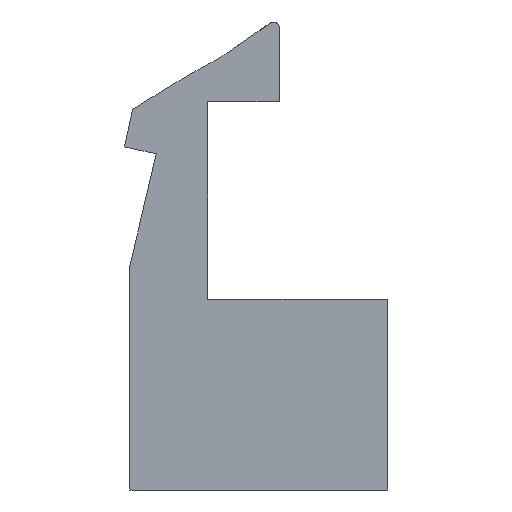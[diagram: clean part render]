
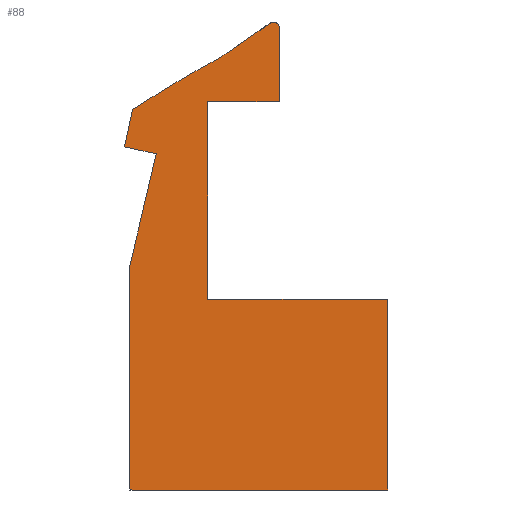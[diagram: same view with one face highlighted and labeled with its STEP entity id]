
A CAD part, front view. The second image highlights one B-rep face of the part: STEP entity #88.
In plain terms, the highlighted planar face has unit normal (0, -1, 0).
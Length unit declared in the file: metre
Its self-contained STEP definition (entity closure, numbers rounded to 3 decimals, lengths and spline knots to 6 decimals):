
#88=ADVANCED_FACE('12:6837',(#170),#171,.F.);
#170=FACE_OUTER_BOUND('',#1109,.T.);
#171=PLANE('',#1110);
#1109=EDGE_LOOP('',(#1387,#1388,#1389,#1390,#1391,#1392,#1393,#1394,#1395,#1396,#1397,#1398,#1399,#1400,#1401,#1402,#1403,#1404,#1405));
#1110=AXIS2_PLACEMENT_3D('',#1406,#1407,#1408);
#1387=ORIENTED_EDGE('',*,*,#1453,.F.);
#1388=ORIENTED_EDGE('',*,*,#1511,.T.);
#1389=ORIENTED_EDGE('',*,*,#1514,.F.);
#1390=ORIENTED_EDGE('',*,*,#1507,.F.);
#1391=ORIENTED_EDGE('',*,*,#1500,.T.);
#1392=ORIENTED_EDGE('',*,*,#1542,.F.);
#1393=ORIENTED_EDGE('',*,*,#1449,.F.);
#1394=ORIENTED_EDGE('',*,*,#1546,.F.);
#1395=ORIENTED_EDGE('',*,*,#1549,.F.);
#1396=ORIENTED_EDGE('',*,*,#1551,.F.);
#1397=ORIENTED_EDGE('',*,*,#1553,.F.);
#1398=ORIENTED_EDGE('',*,*,#1532,.F.);
#1399=ORIENTED_EDGE('',*,*,#1528,.T.);
#1400=ORIENTED_EDGE('',*,*,#1524,.F.);
#1401=ORIENTED_EDGE('',*,*,#1520,.F.);
#1402=ORIENTED_EDGE('',*,*,#1554,.F.);
#1403=ORIENTED_EDGE('',*,*,#1541,.F.);
#1404=ORIENTED_EDGE('',*,*,#1536,.T.);
#1405=ORIENTED_EDGE('',*,*,#1533,.F.);
#1406=CARTESIAN_POINT('',(0.000691,-0.01,0.018046));
#1407=DIRECTION('',(0.,1.0,0.));
#1408=DIRECTION('',(0.214,0.,0.977));
#1449=EDGE_CURVE('12:6918',#1562,#1558,#1564,.F.);
#1453=EDGE_CURVE('12:6894',#1570,#1566,#1572,.F.);
#1500=EDGE_CURVE('12:6915',#1655,#1653,#1656,.F.);
#1507=EDGE_CURVE('12:6912',#1655,#1664,#1665,.F.);
#1511=EDGE_CURVE('12:6906',#1570,#1668,#1670,.F.);
#1514=EDGE_CURVE('12:6909',#1664,#1668,#1674,.T.);
#1520=EDGE_CURVE('12:6942',#1682,#1684,#1685,.T.);
#1524=EDGE_CURVE('12:6939',#1684,#1690,#1691,.T.);
#1528=EDGE_CURVE('12:6936',#1694,#1690,#1697,.T.);
#1532=EDGE_CURVE('12:6933',#1694,#1700,#1703,.T.);
#1533=EDGE_CURVE('12:6894',#1566,#1704,#1705,.F.);
#1536=EDGE_CURVE('12:6951',#1709,#1704,#1710,.F.);
#1541=EDGE_CURVE('12:6948',#1709,#1715,#1718,.F.);
#1542=EDGE_CURVE('12:6918',#1558,#1653,#1719,.F.);
#1546=EDGE_CURVE('12:6921',#1723,#1562,#1725,.F.);
#1549=EDGE_CURVE('12:6924',#1728,#1723,#1730,.T.);
#1551=EDGE_CURVE('12:6927',#1731,#1728,#1734,.F.);
#1553=EDGE_CURVE('12:6930',#1700,#1731,#1736,.T.);
#1554=EDGE_CURVE('12:6945',#1715,#1682,#1737,.F.);
#1558=VERTEX_POINT('',#1741);
#1562=VERTEX_POINT('',#1746);
#1564=CIRCLE('',#1749,0.0535);
#1566=VERTEX_POINT('',#1751);
#1570=VERTEX_POINT('',#1756);
#1572=CIRCLE('',#1759,0.0003);
#1653=VERTEX_POINT('',#1948);
#1655=VERTEX_POINT('',#1951);
#1656=CIRCLE('',#1952,0.002);
#1664=VERTEX_POINT('',#1966);
#1665=CIRCLE('',#1967,0.006);
#1668=VERTEX_POINT('',#1972);
#1670=LINE('',#1975,#1976);
#1674=CIRCLE('',#1982,0.006);
#1682=VERTEX_POINT('',#1992);
#1684=VERTEX_POINT('',#1995);
#1685=LINE('',#1996,#1997);
#1690=VERTEX_POINT('',#2004);
#1691=LINE('',#2005,#2006);
#1694=VERTEX_POINT('',#2010);
#1697=LINE('',#2015,#2016);
#1700=VERTEX_POINT('',#2019);
#1703=LINE('',#2024,#2025);
#1704=VERTEX_POINT('',#2026);
#1705=CIRCLE('',#2027,0.0003);
#1709=VERTEX_POINT('',#2032);
#1710=LINE('',#2033,#2034);
#1715=VERTEX_POINT('',#2041);
#1718=LINE('',#2046,#2047);
#1719=CIRCLE('',#2048,0.0535);
#1723=VERTEX_POINT('',#2053);
#1725=LINE('',#2056,#2057);
#1728=VERTEX_POINT('',#2061);
#1730=LINE('',#2064,#2065);
#1731=VERTEX_POINT('',#2066);
#1734=LINE('',#2070,#2071);
#1736=LINE('',#2074,#2075);
#1737=LINE('',#2076,#2077);
#1741=CARTESIAN_POINT('',(0.002793,-0.01,0.021584));
#1746=CARTESIAN_POINT('',(0.000989,-0.01,0.020483));
#1749=AXIS2_PLACEMENT_3D('',#2087,#2088,#2089);
#1751=CARTESIAN_POINT('',(0.007659,-0.01,0.024499));
#1756=CARTESIAN_POINT('',(0.007348,-0.01,0.024479));
#1759=AXIS2_PLACEMENT_3D('',#2095,#2096,#2097);
#1948=CARTESIAN_POINT('',(0.004638,-0.01,0.022612));
#1951=CARTESIAN_POINT('',(0.004872,-0.01,0.022758));
#1952=AXIS2_PLACEMENT_3D('',#2159,#2160,#2161);
#1966=CARTESIAN_POINT('',(0.005165,-0.01,0.022957));
#1967=AXIS2_PLACEMENT_3D('',#2168,#2169,#2170);
#1972=CARTESIAN_POINT('',(0.005379,-0.01,0.0231));
#1975=CARTESIAN_POINT('',(0.003839,-0.01,0.022023));
#1976=VECTOR('',#2174,1.0);
#1982=AXIS2_PLACEMENT_3D('',#2177,#2178,#2179);
#1992=CARTESIAN_POINT('',(0.004069,-0.01,0.01));
#1995=CARTESIAN_POINT('',(0.0135,-0.01,0.01));
#1996=CARTESIAN_POINT('',(0.005,-0.01,0.01));
#1997=VECTOR('',#2189,1.0);
#2004=CARTESIAN_POINT('',(0.0135,-0.01,0.0));
#2005=CARTESIAN_POINT('',(0.0135,-0.01,0.0));
#2006=VECTOR('',#2195,1.0);
#2010=CARTESIAN_POINT('',(0.,-0.01,0.0));
#2015=CARTESIAN_POINT('',(0.0,-0.01,0.0));
#2016=VECTOR('',#2199,1.0);
#2019=CARTESIAN_POINT('',(0.,-0.01,0.011791));
#2024=CARTESIAN_POINT('',(0.0,-0.01,0.0));
#2025=VECTOR('',#2205,1.0);
#2026=CARTESIAN_POINT('',(0.00782,-0.01,0.024233));
#2027=AXIS2_PLACEMENT_3D('',#2206,#2207,#2208);
#2032=CARTESIAN_POINT('',(0.00782,-0.01,0.02035));
#2033=CARTESIAN_POINT('',(0.00782,-0.01,0.018884));
#2034=VECTOR('',#2213,1.0);
#2041=CARTESIAN_POINT('',(0.004069,-0.01,0.02035));
#2046=CARTESIAN_POINT('',(0.000345,-0.01,0.02035));
#2047=VECTOR('',#2218,1.0);
#2048=AXIS2_PLACEMENT_3D('',#2219,#2220,#2221);
#2053=CARTESIAN_POINT('',(0.000138,-0.01,0.019941));
#2056=CARTESIAN_POINT('',(0.004023,-0.01,0.022418));
#2057=VECTOR('',#2227,1.);
#2061=CARTESIAN_POINT('',(-0.00029,-0.01,0.017987));
#2064=CARTESIAN_POINT('',(-0.000154,-0.01,0.018606));
#2065=VECTOR('',#2230,1.0);
#2066=CARTESIAN_POINT('',(0.001379,-0.01,0.017621));
#2070=CARTESIAN_POINT('',(0.000555,-0.01,0.017802));
#2071=VECTOR('',#2232,1.0);
#2074=CARTESIAN_POINT('',(0.,-0.01,0.011791));
#2075=VECTOR('',#2234,1.);
#2076=CARTESIAN_POINT('',(0.004069,-0.01,0.019273));
#2077=VECTOR('',#2235,0.01);
#2087=CARTESIAN_POINT('',(0.029755,-0.01,-0.024625));
#2088=DIRECTION('',(0.,-1.0,0.));
#2089=DIRECTION('',(-0.504,0.,0.864));
#2095=CARTESIAN_POINT('',(0.00752,-0.01,0.024233));
#2096=DIRECTION('',(0.,-1.0,0.));
#2097=DIRECTION('',(0.462,0.,0.887));
#2159=CARTESIAN_POINT('',(0.003699,-0.01,0.024378));
#2160=DIRECTION('',(0.,-1.0,0.));
#2161=DIRECTION('',(-0.192,0.,0.981));
#2168=CARTESIAN_POINT('',(0.008391,-0.01,0.017899));
#2169=DIRECTION('',(0.,-1.0,0.));
#2170=DIRECTION('',(-0.586,0.,0.81));
#2174=DIRECTION('',(0.819,0.,0.573));
#2177=CARTESIAN_POINT('',(0.001938,-0.01,0.028016));
#2178=DIRECTION('',(0.,-1.0,0.));
#2179=DIRECTION('',(0.668,0.,-0.745));
#2189=DIRECTION('',(1.0,0.0,0.0));
#2195=DIRECTION('',(0.0,0.0,-1.0));
#2199=DIRECTION('',(1.0,0.0,0.0));
#2205=DIRECTION('',(0.0,0.0,1.0));
#2206=CARTESIAN_POINT('',(0.00752,-0.01,0.024233));
#2207=DIRECTION('',(0.,-1.0,0.));
#2208=DIRECTION('',(0.462,0.,0.887));
#2213=DIRECTION('',(0.,0.,-1.0));
#2218=DIRECTION('',(1.0,0.,0.));
#2219=CARTESIAN_POINT('',(0.029755,-0.01,-0.024625));
#2220=DIRECTION('',(0.,-1.0,0.));
#2221=DIRECTION('',(-0.504,0.,0.864));
#2227=DIRECTION('',(-0.843,0.,-0.538));
#2230=DIRECTION('',(0.214,0.,0.977));
#2232=DIRECTION('',(0.977,0.,-0.214));
#2234=DIRECTION('',(0.23,0.0,0.973));
#2235=DIRECTION('',(0.0,0.,1.0));
